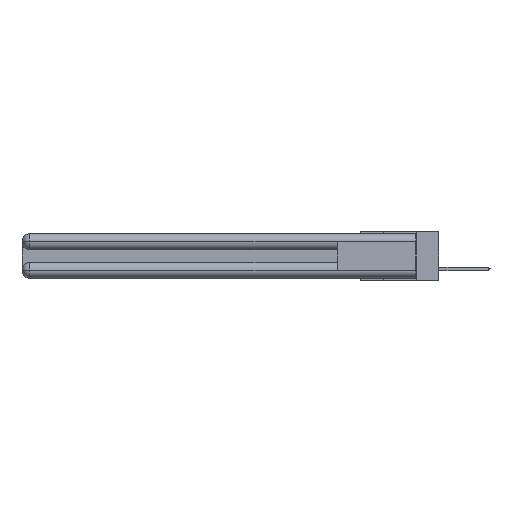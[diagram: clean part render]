
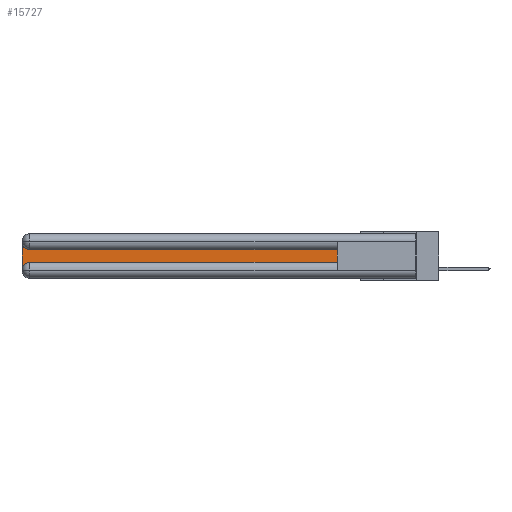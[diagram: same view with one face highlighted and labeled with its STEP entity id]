
A CAD part, left-side view. The second image highlights one B-rep face of the part: STEP entity #15727.
In plain terms, the highlighted planar face has unit normal (-1, 0, 0).
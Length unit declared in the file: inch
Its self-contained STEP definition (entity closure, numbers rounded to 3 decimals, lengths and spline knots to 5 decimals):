
#809 = DIRECTION ( 'NONE',  ( 0., 0., -1. ) ) ;
#1361 = ORIENTED_EDGE ( 'NONE', *, *, #15011, .T. ) ;
#1365 = AXIS2_PLACEMENT_3D ( 'NONE', #18299, #20062, #2684 ) ;
#2185 = DIRECTION ( 'NONE',  ( 0., 0., -1. ) ) ;
#2200 = VERTEX_POINT ( 'NONE', #29664 ) ;
#2684 = DIRECTION ( 'NONE',  ( 0., 0., -1. ) ) ;
#6167 = LINE ( 'NONE', #7397, #27739 ) ;
#6367 = AXIS2_PLACEMENT_3D ( 'NONE', #24168, #26519, #809 ) ;
#6485 = FACE_OUTER_BOUND ( 'NONE', #10664, .T. ) ;
#6842 = CARTESIAN_POINT ( 'NONE',  ( 0.075, 3., -0.1225 ) ) ;
#7397 = CARTESIAN_POINT ( 'NONE',  ( 0.075, 3., -0.2175 ) ) ;
#7513 = DIRECTION ( 'NONE',  ( 0., 0., -1. ) ) ;
#8039 = ORIENTED_EDGE ( 'NONE', *, *, #10963, .T. ) ;
#8204 = LINE ( 'NONE', #25132, #16988 ) ;
#8787 = DIRECTION ( 'NONE',  ( 0., -1., 0. ) ) ;
#8999 = VERTEX_POINT ( 'NONE', #10134 ) ;
#10134 = CARTESIAN_POINT ( 'NONE',  ( 0.075, 3., -0.0625 ) ) ;
#10664 = EDGE_LOOP ( 'NONE', ( #13133, #8039, #1361, #27791, #12403, #15369 ) ) ;
#10679 = LINE ( 'NONE', #16636, #19459 ) ;
#10963 = EDGE_CURVE ( 'NONE', #12570, #8999, #15723, .T. ) ;
#12403 = ORIENTED_EDGE ( 'NONE', *, *, #14060, .T. ) ;
#12570 = VERTEX_POINT ( 'NONE', #22408 ) ;
#13114 = DIRECTION ( 'NONE',  ( 0., 1., 0. ) ) ;
#13133 = ORIENTED_EDGE ( 'NONE', *, *, #27469, .T. ) ;
#13804 = PLANE ( 'NONE',  #15593 ) ;
#14060 = EDGE_CURVE ( 'NONE', #25492, #18342, #8204, .T. ) ;
#14405 = DIRECTION ( 'NONE',  ( 0., 0., 1. ) ) ;
#15011 = EDGE_CURVE ( 'NONE', #8999, #22588, #6167, .T. ) ;
#15053 = EDGE_CURVE ( 'NONE', #22588, #25492, #15321, .T. ) ;
#15066 = CARTESIAN_POINT ( 'NONE',  ( 0.075, 2.94, -0.2175 ) ) ;
#15321 = CIRCLE ( 'NONE', #6367, 0.06 ) ;
#15369 = ORIENTED_EDGE ( 'NONE', *, *, #28224, .T. ) ;
#15593 = AXIS2_PLACEMENT_3D ( 'NONE', #6842, #16232, #2185 ) ;
#15723 = CIRCLE ( 'NONE', #1365, 0.06 ) ;
#15727 = ADVANCED_FACE ( 'NONE', ( #6485 ), #13804, .F. ) ;
#16232 = DIRECTION ( 'NONE',  ( 1., 0., 0. ) ) ;
#16636 = CARTESIAN_POINT ( 'NONE',  ( 0.075, 0.6, -0.2175 ) ) ;
#16988 = VECTOR ( 'NONE', #8787, 39.37008 ) ;
#18299 = CARTESIAN_POINT ( 'NONE',  ( 0.075, 2.94, -0.0625 ) ) ;
#18342 = VERTEX_POINT ( 'NONE', #24557 ) ;
#19459 = VECTOR ( 'NONE', #14405, 39.37008 ) ;
#20062 = DIRECTION ( 'NONE',  ( 1., 0., 0. ) ) ;
#22408 = CARTESIAN_POINT ( 'NONE',  ( 0.075, 2.94, -0.1225 ) ) ;
#22588 = VERTEX_POINT ( 'NONE', #25766 ) ;
#24168 = CARTESIAN_POINT ( 'NONE',  ( 0.075, 2.94, -0.2775 ) ) ;
#24303 = LINE ( 'NONE', #27114, #25370 ) ;
#24557 = CARTESIAN_POINT ( 'NONE',  ( 0.075, 0.6, -0.2175 ) ) ;
#25132 = CARTESIAN_POINT ( 'NONE',  ( 0.075, 0.6, -0.2175 ) ) ;
#25370 = VECTOR ( 'NONE', #13114, 39.37008 ) ;
#25492 = VERTEX_POINT ( 'NONE', #15066 ) ;
#25766 = CARTESIAN_POINT ( 'NONE',  ( 0.075, 3., -0.2775 ) ) ;
#26519 = DIRECTION ( 'NONE',  ( 1., 0., 0. ) ) ;
#27114 = CARTESIAN_POINT ( 'NONE',  ( 0.075, 0.6, -0.1225 ) ) ;
#27469 = EDGE_CURVE ( 'NONE', #2200, #12570, #24303, .T. ) ;
#27739 = VECTOR ( 'NONE', #7513, 39.37008 ) ;
#27791 = ORIENTED_EDGE ( 'NONE', *, *, #15053, .T. ) ;
#28224 = EDGE_CURVE ( 'NONE', #18342, #2200, #10679, .T. ) ;
#29664 = CARTESIAN_POINT ( 'NONE',  ( 0.075, 0.6, -0.1225 ) ) ;
